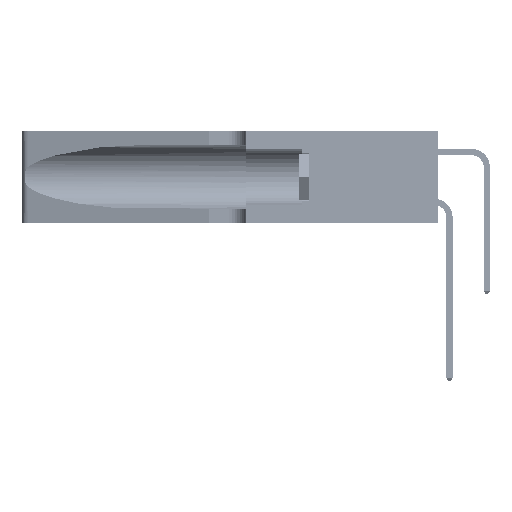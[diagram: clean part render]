
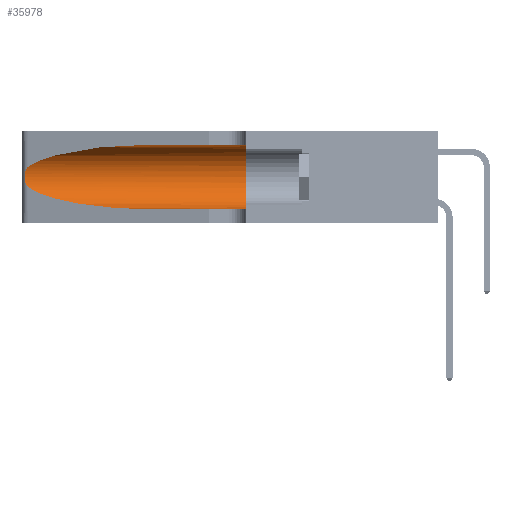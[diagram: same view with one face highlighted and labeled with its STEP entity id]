
A CAD part, left-side view. The second image highlights one B-rep face of the part: STEP entity #35978.
In plain terms, the highlighted cylindrical face has radius 3.308 mm (diameter 6.617 mm), a partial arc.
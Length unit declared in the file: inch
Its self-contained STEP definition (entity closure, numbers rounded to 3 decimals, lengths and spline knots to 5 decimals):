
#877 = CARTESIAN_POINT ( 'NONE',  ( 0.25555, 1.22994, 0.2215 ) ) ;
#1217 = CARTESIAN_POINT ( 'NONE',  ( 0.25487, 1.22718, 0.22369 ) ) ;
#1700 = CARTESIAN_POINT ( 'NONE',  ( 0.25487, 1.22718, 0.22369 ) ) ;
#1852 = CARTESIAN_POINT ( 'NONE',  ( 0.1305, 0.72297, 0.31525 ) ) ;
#2315 = CARTESIAN_POINT ( 'NONE',  ( 0.25487, 1.22718, 0.22369 ) ) ;
#2629 = CARTESIAN_POINT ( 'NONE',  ( 0.1305, 1.61858, 0.185 ) ) ;
#4561 = CARTESIAN_POINT ( 'NONE',  ( 0.2373, 1.15595, 0.08982 ) ) ;
#4875 = CARTESIAN_POINT ( 'NONE',  ( 0.25854, 1.2359, 0.20912 ) ) ;
#4985 = AXIS2_PLACEMENT_3D ( 'NONE', #42358, #28248, #32388 ) ;
#8169 = ORIENTED_EDGE ( 'NONE', *, *, #42145, .T. ) ;
#8722 = CARTESIAN_POINT ( 'NONE',  ( 0.25787, 1.23484, 0.2124 ) ) ;
#9788 = EDGE_CURVE ( 'NONE', #30147, #31523, #15755, .T. ) ;
#10001 = VERTEX_POINT ( 'NONE', #47236 ) ;
#10691 = VECTOR ( 'NONE', #41645, 39.37008 ) ;
#11067 = CARTESIAN_POINT ( 'NONE',  ( 0.1305, 1.61858, 0.05475 ) ) ;
#12376 = CARTESIAN_POINT ( 'NONE',  ( 0.25487, 1.22718, 0.14631 ) ) ;
#12538 = CARTESIAN_POINT ( 'NONE',  ( 0.26017, 1.23833, 0.17102 ) ) ;
#13050 = ORIENTED_EDGE ( 'NONE', *, *, #30693, .T. ) ;
#14199 = EDGE_CURVE ( 'NONE', #24267, #35743, #19448, .T. ) ;
#14915 = CARTESIAN_POINT ( 'NONE',  ( 0.1305, 0.35, 0.05475 ) ) ;
#15755 = CIRCLE ( 'NONE', #4985, 0.13025 ) ;
#16172 = CARTESIAN_POINT ( 'NONE',  ( 0.25789, 1.23486, 0.15765 ) ) ;
#17316 = EDGE_LOOP ( 'NONE', ( #13050, #18417, #22484, #8169, #35030, #33910 ) ) ;
#18417 = ORIENTED_EDGE ( 'NONE', *, *, #30478, .T. ) ;
#19448 =( BOUNDED_CURVE ( )  B_SPLINE_CURVE ( 3, ( #12376, #4561, #31512, #20188 ),
 .UNSPECIFIED., .F., .F. ) 
 B_SPLINE_CURVE_WITH_KNOTS ( ( 4, 4 ),
 ( 3.44316, 4.71239 ),
 .UNSPECIFIED. ) 
 CURVE ( )  GEOMETRIC_REPRESENTATION_ITEM ( )  RATIONAL_B_SPLINE_CURVE ( ( 1., 0.87, 0.87, 1. ) ) 
 REPRESENTATION_ITEM ( '' )  );
#19709 = VECTOR ( 'NONE', #24796, 39.37008 ) ;
#20180 = CARTESIAN_POINT ( 'NONE',  ( 0.25487, 1.22718, 0.14631 ) ) ;
#20183 = CARTESIAN_POINT ( 'NONE',  ( 0.25487, 1.22718, 0.14631 ) ) ;
#20188 = CARTESIAN_POINT ( 'NONE',  ( 0.1305, 0.72297, 0.05475 ) ) ;
#20291 = FACE_OUTER_BOUND ( 'NONE', #17316, .T. ) ;
#20351 = AXIS2_PLACEMENT_3D ( 'NONE', #2629, #37240, #44876 ) ;
#21376 = CARTESIAN_POINT ( 'NONE',  ( 0.1305, 0.35, 0.31525 ) ) ;
#22484 = ORIENTED_EDGE ( 'NONE', *, *, #14199, .T. ) ;
#23686 = CARTESIAN_POINT ( 'NONE',  ( 0.26075, 1.23896, 0.178 ) ) ;
#24061 = B_SPLINE_CURVE_WITH_KNOTS ( 'NONE', 3,
 ( #1217, #877, #46477, #8722, #4875, #39006, #35637, #23686, #12538, #43133, #16172, #39327, #42799, #20180 ),
 .UNSPECIFIED., .F., .F.,
 ( 4, 2, 2, 2, 2, 2, 4 ),
 ( 0., 0.00027, 0.00053, 0.00107, 0.0016, 0.00187, 0.00214 ),
 .UNSPECIFIED. ) ;
#24267 = VERTEX_POINT ( 'NONE', #20183 ) ;
#24513 = CARTESIAN_POINT ( 'NONE',  ( 0.2373, 1.15595, 0.28018 ) ) ;
#24796 = DIRECTION ( 'NONE',  ( 0., -1., 0. ) ) ;
#24845 = CARTESIAN_POINT ( 'NONE',  ( 0.18966, 0.96281, 0.31525 ) ) ;
#24956 = CARTESIAN_POINT ( 'NONE',  ( 0.1305, 1.61858, 0.31525 ) ) ;
#25933 = CARTESIAN_POINT ( 'NONE',  ( 0.1305, 0.72297, 0.05475 ) ) ;
#28248 = DIRECTION ( 'NONE',  ( 0., 1., 0. ) ) ;
#30147 = VERTEX_POINT ( 'NONE', #21376 ) ;
#30478 = EDGE_CURVE ( 'NONE', #39266, #24267, #24061, .T. ) ;
#30693 = EDGE_CURVE ( 'NONE', #10001, #39266, #39587, .T. ) ;
#31512 = CARTESIAN_POINT ( 'NONE',  ( 0.18966, 0.96281, 0.05475 ) ) ;
#31523 = VERTEX_POINT ( 'NONE', #14915 ) ;
#32388 = DIRECTION ( 'NONE',  ( 0., 0., 1. ) ) ;
#33865 = LINE ( 'NONE', #11067, #10691 ) ;
#33910 = ORIENTED_EDGE ( 'NONE', *, *, #41158, .F. ) ;
#35030 = ORIENTED_EDGE ( 'NONE', *, *, #9788, .F. ) ;
#35637 = CARTESIAN_POINT ( 'NONE',  ( 0.26075, 1.23896, 0.19203 ) ) ;
#35743 = VERTEX_POINT ( 'NONE', #25933 ) ;
#35978 = ADVANCED_FACE ( 'NONE', ( #20291 ), #45287, .F. ) ;
#36991 = LINE ( 'NONE', #24956, #19709 ) ;
#37240 = DIRECTION ( 'NONE',  ( 0., -1., 0. ) ) ;
#39006 = CARTESIAN_POINT ( 'NONE',  ( 0.26018, 1.23835, 0.19895 ) ) ;
#39266 = VERTEX_POINT ( 'NONE', #2315 ) ;
#39327 = CARTESIAN_POINT ( 'NONE',  ( 0.25639, 1.23186, 0.15144 ) ) ;
#39587 =( BOUNDED_CURVE ( )  B_SPLINE_CURVE ( 3, ( #1852, #24845, #24513, #1700 ),
 .UNSPECIFIED., .F., .F. ) 
 B_SPLINE_CURVE_WITH_KNOTS ( ( 4, 4 ),
 ( 1.5708, 2.84003 ),
 .UNSPECIFIED. ) 
 CURVE ( )  GEOMETRIC_REPRESENTATION_ITEM ( )  RATIONAL_B_SPLINE_CURVE ( ( 1., 0.87, 0.87, 1. ) ) 
 REPRESENTATION_ITEM ( '' )  );
#41158 = EDGE_CURVE ( 'NONE', #10001, #30147, #36991, .T. ) ;
#41645 = DIRECTION ( 'NONE',  ( 0., -1., 0. ) ) ;
#42145 = EDGE_CURVE ( 'NONE', #35743, #31523, #33865, .T. ) ;
#42358 = CARTESIAN_POINT ( 'NONE',  ( 0.1305, 0.35, 0.185 ) ) ;
#42799 = CARTESIAN_POINT ( 'NONE',  ( 0.25555, 1.22993, 0.14849 ) ) ;
#43133 = CARTESIAN_POINT ( 'NONE',  ( 0.25856, 1.23593, 0.16098 ) ) ;
#44876 = DIRECTION ( 'NONE',  ( 0., 0., -1. ) ) ;
#45287 = CYLINDRICAL_SURFACE ( 'NONE', #20351, 0.13025 ) ;
#46477 = CARTESIAN_POINT ( 'NONE',  ( 0.25639, 1.23184, 0.21858 ) ) ;
#47236 = CARTESIAN_POINT ( 'NONE',  ( 0.1305, 0.72297, 0.31525 ) ) ;
